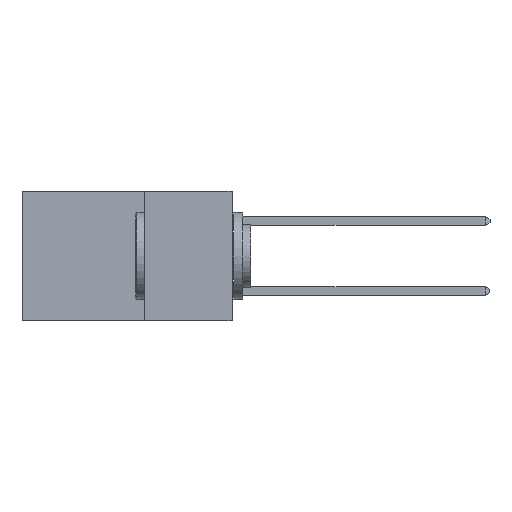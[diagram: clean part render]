
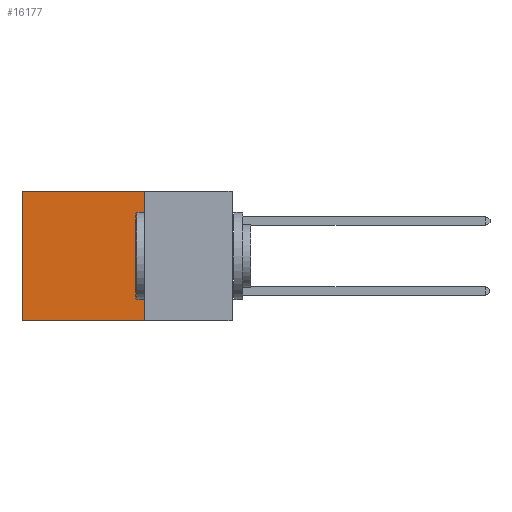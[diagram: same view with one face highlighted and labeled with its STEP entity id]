
A CAD part, left-side view. The second image highlights one B-rep face of the part: STEP entity #16177.
In plain terms, the highlighted planar face has unit normal (-1, 0, 0).
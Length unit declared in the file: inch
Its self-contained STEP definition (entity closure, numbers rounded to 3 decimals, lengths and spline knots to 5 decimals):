
#253 = EDGE_LOOP ( 'NONE', ( #9860, #6007, #15716, #2166 ) ) ;
#455 = DIRECTION ( 'NONE',  ( 1., 0., 0. ) ) ;
#472 = VECTOR ( 'NONE', #11981, 39.37008 ) ;
#830 = VERTEX_POINT ( 'NONE', #8675 ) ;
#1538 = EDGE_CURVE ( 'NONE', #11929, #9808, #6481, .T. ) ;
#1750 = CARTESIAN_POINT ( 'NONE',  ( 0.2875, 0.6, 0. ) ) ;
#2166 = ORIENTED_EDGE ( 'NONE', *, *, #3921, .T. ) ;
#2393 = LINE ( 'NONE', #15634, #15528 ) ;
#3133 = DIRECTION ( 'NONE',  ( 0., 1., 0. ) ) ;
#3261 = VECTOR ( 'NONE', #12206, 39.37008 ) ;
#3712 = CARTESIAN_POINT ( 'NONE',  ( 0.2875, 0.6, -0.37 ) ) ;
#3921 = EDGE_CURVE ( 'NONE', #830, #8484, #2393, .T. ) ;
#4247 = AXIS2_PLACEMENT_3D ( 'NONE', #8223, #455, #9530 ) ;
#5563 = CARTESIAN_POINT ( 'NONE',  ( 0.2875, 0.25, -0.37 ) ) ;
#5596 = PLANE ( 'NONE',  #4247 ) ;
#6007 = ORIENTED_EDGE ( 'NONE', *, *, #1538, .F. ) ;
#6481 = LINE ( 'NONE', #5563, #15797 ) ;
#6659 = LINE ( 'NONE', #14453, #3261 ) ;
#8223 = CARTESIAN_POINT ( 'NONE',  ( 0.2875, 0.25, 0. ) ) ;
#8287 = FACE_OUTER_BOUND ( 'NONE', #253, .T. ) ;
#8484 = VERTEX_POINT ( 'NONE', #15395 ) ;
#8675 = CARTESIAN_POINT ( 'NONE',  ( 0.2875, 0.25, 0. ) ) ;
#8687 = EDGE_CURVE ( 'NONE', #8484, #9808, #11524, .T. ) ;
#9530 = DIRECTION ( 'NONE',  ( 0., 0., -1. ) ) ;
#9808 = VERTEX_POINT ( 'NONE', #3712 ) ;
#9860 = ORIENTED_EDGE ( 'NONE', *, *, #8687, .T. ) ;
#11524 = LINE ( 'NONE', #1750, #472 ) ;
#11929 = VERTEX_POINT ( 'NONE', #14878 ) ;
#11981 = DIRECTION ( 'NONE',  ( 0., 0., -1. ) ) ;
#12206 = DIRECTION ( 'NONE',  ( 0., 0., -1. ) ) ;
#14312 = EDGE_CURVE ( 'NONE', #830, #11929, #6659, .T. ) ;
#14453 = CARTESIAN_POINT ( 'NONE',  ( 0.2875, 0.25, 0. ) ) ;
#14878 = CARTESIAN_POINT ( 'NONE',  ( 0.2875, 0.25, -0.37 ) ) ;
#15395 = CARTESIAN_POINT ( 'NONE',  ( 0.2875, 0.6, 0. ) ) ;
#15528 = VECTOR ( 'NONE', #15577, 39.37008 ) ;
#15577 = DIRECTION ( 'NONE',  ( 0., 1., 0. ) ) ;
#15634 = CARTESIAN_POINT ( 'NONE',  ( 0.2875, 0.25, 0. ) ) ;
#15716 = ORIENTED_EDGE ( 'NONE', *, *, #14312, .F. ) ;
#15797 = VECTOR ( 'NONE', #3133, 39.37008 ) ;
#16177 = ADVANCED_FACE ( 'NONE', ( #8287 ), #5596, .F. ) ;
